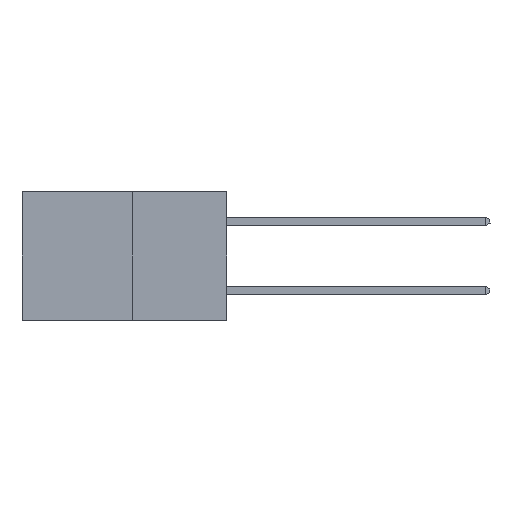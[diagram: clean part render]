
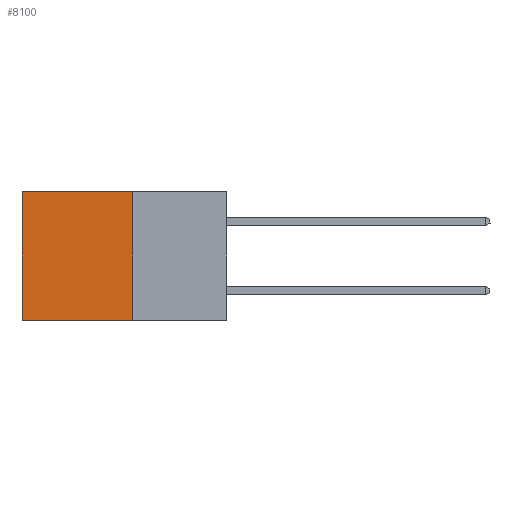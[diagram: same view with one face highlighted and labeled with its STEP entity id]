
A CAD part, left-side view. The second image highlights one B-rep face of the part: STEP entity #8100.
In plain terms, the highlighted planar face has unit normal (-1, 0, 0).
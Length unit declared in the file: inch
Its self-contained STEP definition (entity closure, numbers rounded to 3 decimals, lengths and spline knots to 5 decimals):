
#1043 = DIRECTION ( 'NONE',  ( 0., 0., -1. ) ) ;
#1540 = DIRECTION ( 'NONE',  ( 0., 0., -1. ) ) ;
#1886 = DIRECTION ( 'NONE',  ( 0., 1., 0. ) ) ;
#3052 = EDGE_LOOP ( 'NONE', ( #7767, #10261, #6225, #9374 ) ) ;
#3388 = LINE ( 'NONE', #3391, #5114 ) ;
#3391 = CARTESIAN_POINT ( 'NONE',  ( 0.277, 0.27, -0.37 ) ) ;
#3616 = CARTESIAN_POINT ( 'NONE',  ( 0.277, 0.27, -0.37 ) ) ;
#3872 = VECTOR ( 'NONE', #1043, 39.37008 ) ;
#3927 = CARTESIAN_POINT ( 'NONE',  ( 0.277, 0.59, 0. ) ) ;
#4246 = EDGE_CURVE ( 'NONE', #8523, #7802, #10579, .T. ) ;
#4545 = VERTEX_POINT ( 'NONE', #9890 ) ;
#4856 = CARTESIAN_POINT ( 'NONE',  ( 0.277, 0.27, 0. ) ) ;
#5033 = EDGE_CURVE ( 'NONE', #8605, #4545, #10580, .T. ) ;
#5114 = VECTOR ( 'NONE', #10148, 39.37008 ) ;
#5870 = PLANE ( 'NONE',  #7796 ) ;
#6130 = LINE ( 'NONE', #7920, #8387 ) ;
#6225 = ORIENTED_EDGE ( 'NONE', *, *, #5033, .F. ) ;
#6548 = DIRECTION ( 'NONE',  ( 0., 0., -1. ) ) ;
#6747 = DIRECTION ( 'NONE',  ( 1., 0., 0. ) ) ;
#7729 = CARTESIAN_POINT ( 'NONE',  ( 0.277, 0.59, -0.37 ) ) ;
#7767 = ORIENTED_EDGE ( 'NONE', *, *, #4246, .T. ) ;
#7796 = AXIS2_PLACEMENT_3D ( 'NONE', #8400, #6747, #1540 ) ;
#7802 = VERTEX_POINT ( 'NONE', #9504 ) ;
#7920 = CARTESIAN_POINT ( 'NONE',  ( 0.277, 0.27, 0. ) ) ;
#8100 = ADVANCED_FACE ( 'NONE', ( #9864 ), #5870, .F. ) ;
#8148 = EDGE_CURVE ( 'NONE', #4545, #7802, #3388, .T. ) ;
#8387 = VECTOR ( 'NONE', #1886, 39.37008 ) ;
#8400 = CARTESIAN_POINT ( 'NONE',  ( 0.277, 0.27, -0.37 ) ) ;
#8523 = VERTEX_POINT ( 'NONE', #3927 ) ;
#8605 = VERTEX_POINT ( 'NONE', #4856 ) ;
#9374 = ORIENTED_EDGE ( 'NONE', *, *, #10319, .T. ) ;
#9504 = CARTESIAN_POINT ( 'NONE',  ( 0.277, 0.59, -0.37 ) ) ;
#9864 = FACE_OUTER_BOUND ( 'NONE', #3052, .T. ) ;
#9890 = CARTESIAN_POINT ( 'NONE',  ( 0.277, 0.27, -0.37 ) ) ;
#10044 = VECTOR ( 'NONE', #6548, 39.37008 ) ;
#10148 = DIRECTION ( 'NONE',  ( 0., 1., 0. ) ) ;
#10261 = ORIENTED_EDGE ( 'NONE', *, *, #8148, .F. ) ;
#10319 = EDGE_CURVE ( 'NONE', #8605, #8523, #6130, .T. ) ;
#10579 = LINE ( 'NONE', #7729, #10044 ) ;
#10580 = LINE ( 'NONE', #3616, #3872 ) ;
